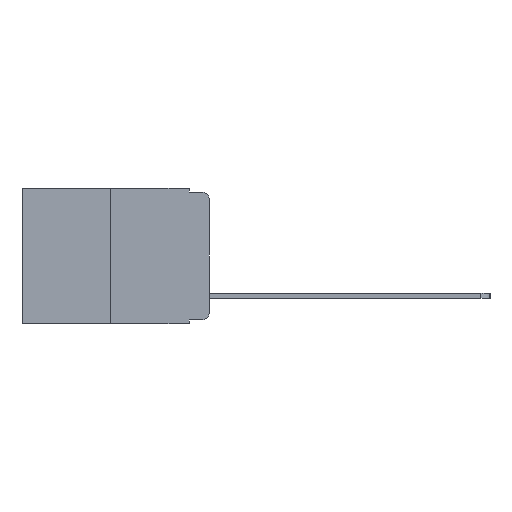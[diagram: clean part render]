
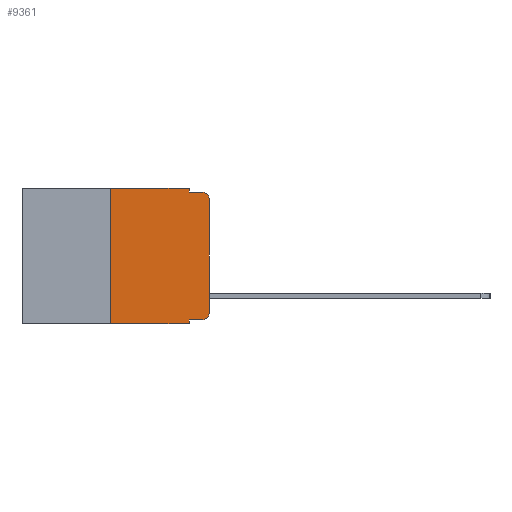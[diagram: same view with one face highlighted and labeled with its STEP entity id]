
A CAD part, left-side view. The second image highlights one B-rep face of the part: STEP entity #9361.
In plain terms, the highlighted planar face has unit normal (-1, 0, 0).
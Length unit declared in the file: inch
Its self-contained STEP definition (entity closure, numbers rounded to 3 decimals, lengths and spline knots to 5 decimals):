
#167 = ORIENTED_EDGE ( 'NONE', *, *, #9413, .F. ) ;
#819 = DIRECTION ( 'NONE',  ( -1., 0., 0. ) ) ;
#976 = EDGE_CURVE ( 'NONE', #9391, #10996, #17291, .T. ) ;
#1128 = LINE ( 'NONE', #18589, #4639 ) ;
#1130 = LINE ( 'NONE', #2932, #5715 ) ;
#1712 = FACE_OUTER_BOUND ( 'NONE', #4807, .T. ) ;
#1883 = VERTEX_POINT ( 'NONE', #13721 ) ;
#2128 = CARTESIAN_POINT ( 'NONE',  ( 0., 0.473, 0. ) ) ;
#2412 = CARTESIAN_POINT ( 'NONE',  ( 0., 0.051, 0. ) ) ;
#2737 = CARTESIAN_POINT ( 'NONE',  ( 0., 0.02, -0.333 ) ) ;
#2932 = CARTESIAN_POINT ( 'NONE',  ( 0., 0., 0. ) ) ;
#3042 = ORIENTED_EDGE ( 'NONE', *, *, #3382, .T. ) ;
#3359 = VECTOR ( 'NONE', #15583, 39.37008 ) ;
#3382 = EDGE_CURVE ( 'NONE', #17860, #10996, #18327, .T. ) ;
#3447 = ORIENTED_EDGE ( 'NONE', *, *, #14227, .F. ) ;
#4271 = LINE ( 'NONE', #6300, #8176 ) ;
#4639 = VECTOR ( 'NONE', #20072, 39.37008 ) ;
#4807 = EDGE_LOOP ( 'NONE', ( #5055, #14221, #167, #18648, #3447, #5822, #3042, #14624, #19956, #13515 ) ) ;
#4904 = CARTESIAN_POINT ( 'NONE',  ( 0., 0.051, 0. ) ) ;
#5055 = ORIENTED_EDGE ( 'NONE', *, *, #20612, .T. ) ;
#5134 = CARTESIAN_POINT ( 'NONE',  ( 0., 0., -0.313 ) ) ;
#5447 = VECTOR ( 'NONE', #7884, 39.37008 ) ;
#5630 = CARTESIAN_POINT ( 'NONE',  ( 0., 0.02, -0.313 ) ) ;
#5715 = VECTOR ( 'NONE', #14442, 39.37008 ) ;
#5822 = ORIENTED_EDGE ( 'NONE', *, *, #16010, .F. ) ;
#6300 = CARTESIAN_POINT ( 'NONE',  ( 0., 0.473, 0. ) ) ;
#6366 = CARTESIAN_POINT ( 'NONE',  ( 0., 0.051, -0.01 ) ) ;
#6458 = DIRECTION ( 'NONE',  ( 0., 0., 1. ) ) ;
#6564 = CARTESIAN_POINT ( 'NONE',  ( 0., 0.051, 0. ) ) ;
#7314 = DIRECTION ( 'NONE',  ( 0., 0., -1. ) ) ;
#7640 = AXIS2_PLACEMENT_3D ( 'NONE', #2128, #8871, #19923 ) ;
#7770 = CARTESIAN_POINT ( 'NONE',  ( 0., 0.25, 0. ) ) ;
#7829 = LINE ( 'NONE', #2412, #3359 ) ;
#7884 = DIRECTION ( 'NONE',  ( 0., -1., 0. ) ) ;
#8176 = VECTOR ( 'NONE', #16071, 39.37008 ) ;
#8871 = DIRECTION ( 'NONE',  ( 1., 0., 0. ) ) ;
#9294 = DIRECTION ( 'NONE',  ( 0., 0., -1. ) ) ;
#9361 = ADVANCED_FACE ( 'NONE', ( #1712 ), #16951, .F. ) ;
#9391 = VERTEX_POINT ( 'NONE', #18513 ) ;
#9413 = EDGE_CURVE ( 'NONE', #15010, #19490, #1128, .T. ) ;
#10247 = CARTESIAN_POINT ( 'NONE',  ( 0., 0.25, -0.343 ) ) ;
#10273 = VERTEX_POINT ( 'NONE', #4904 ) ;
#10898 = CARTESIAN_POINT ( 'NONE',  ( 0., 0.02, -0.03 ) ) ;
#10996 = VERTEX_POINT ( 'NONE', #18014 ) ;
#11039 = DIRECTION ( 'NONE',  ( 0., -1., 0. ) ) ;
#11392 = VECTOR ( 'NONE', #6458, 39.37008 ) ;
#11620 = VERTEX_POINT ( 'NONE', #7770 ) ;
#12246 = EDGE_CURVE ( 'NONE', #1883, #19490, #20622, .T. ) ;
#12404 = CARTESIAN_POINT ( 'NONE',  ( 0., 0.473, -0.343 ) ) ;
#12494 = DIRECTION ( 'NONE',  ( 0., 0., -1. ) ) ;
#13515 = ORIENTED_EDGE ( 'NONE', *, *, #17946, .T. ) ;
#13721 = CARTESIAN_POINT ( 'NONE',  ( 0., 0., -0.03 ) ) ;
#14122 = CARTESIAN_POINT ( 'NONE',  ( 0., 0.051, -0.333 ) ) ;
#14221 = ORIENTED_EDGE ( 'NONE', *, *, #12246, .T. ) ;
#14227 = EDGE_CURVE ( 'NONE', #11620, #10273, #4271, .T. ) ;
#14409 = VECTOR ( 'NONE', #11039, 39.37008 ) ;
#14442 = DIRECTION ( 'NONE',  ( 0., 0., 1. ) ) ;
#14624 = ORIENTED_EDGE ( 'NONE', *, *, #976, .F. ) ;
#15010 = VERTEX_POINT ( 'NONE', #6366 ) ;
#15192 = LINE ( 'NONE', #17782, #11392 ) ;
#15583 = DIRECTION ( 'NONE',  ( 0., 0., -1. ) ) ;
#16010 = EDGE_CURVE ( 'NONE', #17860, #11620, #15192, .T. ) ;
#16071 = DIRECTION ( 'NONE',  ( 0., -1., 0. ) ) ;
#16797 = VECTOR ( 'NONE', #9294, 39.37008 ) ;
#16951 = PLANE ( 'NONE',  #7640 ) ;
#17035 = DIRECTION ( 'NONE',  ( -1., 0., 0. ) ) ;
#17124 = VERTEX_POINT ( 'NONE', #5134 ) ;
#17245 = CIRCLE ( 'NONE', #19151, 0.02 ) ;
#17291 = LINE ( 'NONE', #6564, #16797 ) ;
#17435 = AXIS2_PLACEMENT_3D ( 'NONE', #10898, #819, #12494 ) ;
#17585 = VERTEX_POINT ( 'NONE', #2737 ) ;
#17782 = CARTESIAN_POINT ( 'NONE',  ( 0., 0.25, 0. ) ) ;
#17860 = VERTEX_POINT ( 'NONE', #10247 ) ;
#17946 = EDGE_CURVE ( 'NONE', #17585, #17124, #17245, .T. ) ;
#18014 = CARTESIAN_POINT ( 'NONE',  ( 0., 0.051, -0.343 ) ) ;
#18327 = LINE ( 'NONE', #12404, #5447 ) ;
#18513 = CARTESIAN_POINT ( 'NONE',  ( 0., 0.051, -0.333 ) ) ;
#18589 = CARTESIAN_POINT ( 'NONE',  ( 0., 0.051, -0.01 ) ) ;
#18619 = LINE ( 'NONE', #14122, #14409 ) ;
#18648 = ORIENTED_EDGE ( 'NONE', *, *, #19833, .F. ) ;
#19151 = AXIS2_PLACEMENT_3D ( 'NONE', #5630, #17035, #7314 ) ;
#19299 = CARTESIAN_POINT ( 'NONE',  ( 0., 0.02, -0.01 ) ) ;
#19490 = VERTEX_POINT ( 'NONE', #19299 ) ;
#19833 = EDGE_CURVE ( 'NONE', #10273, #15010, #7829, .T. ) ;
#19909 = EDGE_CURVE ( 'NONE', #9391, #17585, #18619, .T. ) ;
#19923 = DIRECTION ( 'NONE',  ( 0., 0., -1. ) ) ;
#19956 = ORIENTED_EDGE ( 'NONE', *, *, #19909, .T. ) ;
#20072 = DIRECTION ( 'NONE',  ( 0., -1., 0. ) ) ;
#20612 = EDGE_CURVE ( 'NONE', #17124, #1883, #1130, .T. ) ;
#20622 = CIRCLE ( 'NONE', #17435, 0.02 ) ;
